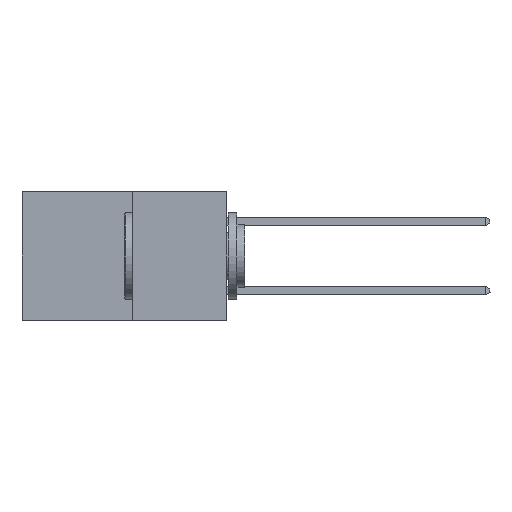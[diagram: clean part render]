
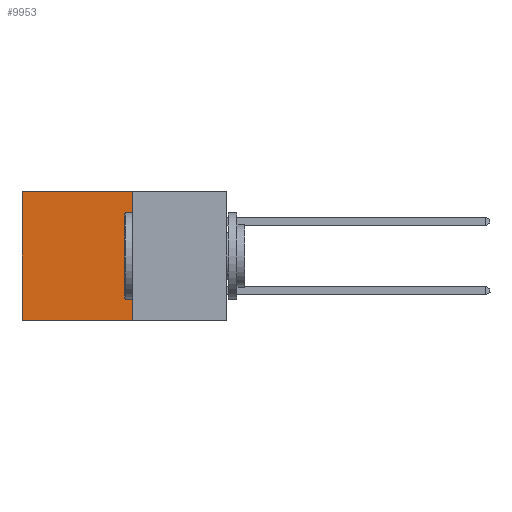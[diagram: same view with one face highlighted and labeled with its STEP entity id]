
A CAD part, left-side view. The second image highlights one B-rep face of the part: STEP entity #9953.
In plain terms, the highlighted planar face has unit normal (-1, 0, 0).
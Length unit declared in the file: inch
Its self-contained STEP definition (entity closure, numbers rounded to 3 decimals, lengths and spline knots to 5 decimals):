
#101 = FACE_OUTER_BOUND ( 'NONE', #8985, .T. ) ;
#291 = VERTEX_POINT ( 'NONE', #6090 ) ;
#529 = DIRECTION ( 'NONE',  ( 0., 1., 0. ) ) ;
#953 = VECTOR ( 'NONE', #7639, 39.37008 ) ;
#1567 = ORIENTED_EDGE ( 'NONE', *, *, #10176, .T. ) ;
#1823 = ORIENTED_EDGE ( 'NONE', *, *, #2370, .F. ) ;
#1966 = VECTOR ( 'NONE', #4113, 39.37008 ) ;
#2370 = EDGE_CURVE ( 'NONE', #3280, #291, #6956, .T. ) ;
#2437 = VERTEX_POINT ( 'NONE', #7273 ) ;
#3022 = CARTESIAN_POINT ( 'NONE',  ( 0.277, 0.27, -0.37 ) ) ;
#3091 = PLANE ( 'NONE',  #6696 ) ;
#3280 = VERTEX_POINT ( 'NONE', #4924 ) ;
#4113 = DIRECTION ( 'NONE',  ( 0., 0., -1. ) ) ;
#4340 = DIRECTION ( 'NONE',  ( 0., 1., 0. ) ) ;
#4404 = CARTESIAN_POINT ( 'NONE',  ( 0.277, 0.27, 0. ) ) ;
#4763 = DIRECTION ( 'NONE',  ( 1., 0., 0. ) ) ;
#4879 = CARTESIAN_POINT ( 'NONE',  ( 0.277, 0.59, -0.37 ) ) ;
#4924 = CARTESIAN_POINT ( 'NONE',  ( 0.277, 0.27, 0. ) ) ;
#5149 = LINE ( 'NONE', #4404, #9132 ) ;
#5924 = ORIENTED_EDGE ( 'NONE', *, *, #9909, .F. ) ;
#6007 = EDGE_CURVE ( 'NONE', #3280, #2437, #5149, .T. ) ;
#6090 = CARTESIAN_POINT ( 'NONE',  ( 0.277, 0.27, -0.37 ) ) ;
#6648 = VECTOR ( 'NONE', #529, 39.37008 ) ;
#6696 = AXIS2_PLACEMENT_3D ( 'NONE', #9543, #4763, #10326 ) ;
#6956 = LINE ( 'NONE', #7614, #953 ) ;
#7147 = LINE ( 'NONE', #3022, #6648 ) ;
#7273 = CARTESIAN_POINT ( 'NONE',  ( 0.277, 0.59, 0. ) ) ;
#7614 = CARTESIAN_POINT ( 'NONE',  ( 0.277, 0.27, -0.37 ) ) ;
#7639 = DIRECTION ( 'NONE',  ( 0., 0., -1. ) ) ;
#8124 = LINE ( 'NONE', #8911, #1966 ) ;
#8911 = CARTESIAN_POINT ( 'NONE',  ( 0.277, 0.59, -0.37 ) ) ;
#8985 = EDGE_LOOP ( 'NONE', ( #1567, #5924, #1823, #10372 ) ) ;
#9132 = VECTOR ( 'NONE', #4340, 39.37008 ) ;
#9543 = CARTESIAN_POINT ( 'NONE',  ( 0.277, 0.27, -0.37 ) ) ;
#9909 = EDGE_CURVE ( 'NONE', #291, #10129, #7147, .T. ) ;
#9953 = ADVANCED_FACE ( 'NONE', ( #101 ), #3091, .F. ) ;
#10129 = VERTEX_POINT ( 'NONE', #4879 ) ;
#10176 = EDGE_CURVE ( 'NONE', #2437, #10129, #8124, .T. ) ;
#10326 = DIRECTION ( 'NONE',  ( 0., 0., -1. ) ) ;
#10372 = ORIENTED_EDGE ( 'NONE', *, *, #6007, .T. ) ;
